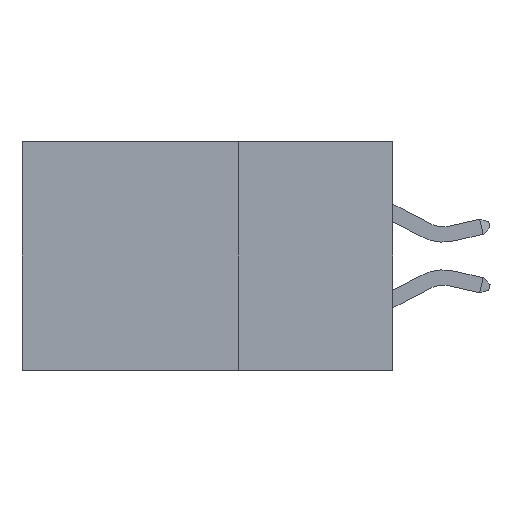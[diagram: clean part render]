
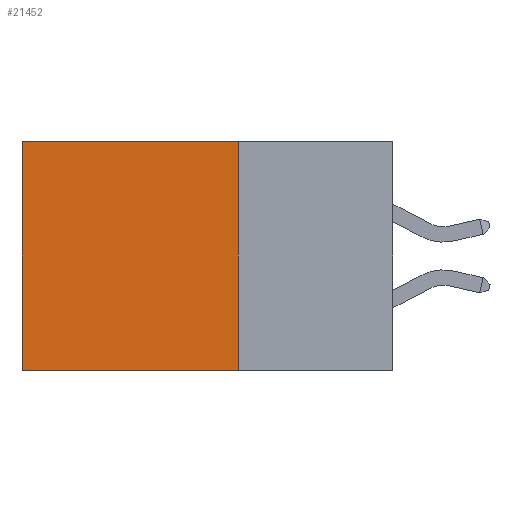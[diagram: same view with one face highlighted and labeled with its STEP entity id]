
A CAD part, left-side view. The second image highlights one B-rep face of the part: STEP entity #21452.
In plain terms, the highlighted planar face has unit normal (-1, 0, 0).
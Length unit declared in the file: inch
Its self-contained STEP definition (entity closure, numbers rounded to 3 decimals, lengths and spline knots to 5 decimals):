
#387 = LINE ( 'NONE', #5251, #19746 ) ;
#1677 = ORIENTED_EDGE ( 'NONE', *, *, #12777, .F. ) ;
#1767 = CARTESIAN_POINT ( 'NONE',  ( 0.2875, 0.6, 0. ) ) ;
#2341 = ORIENTED_EDGE ( 'NONE', *, *, #16443, .T. ) ;
#2818 = CARTESIAN_POINT ( 'NONE',  ( 0.2875, 0.6, -0.37 ) ) ;
#3862 = CARTESIAN_POINT ( 'NONE',  ( 0.2875, 0.25, 0. ) ) ;
#4780 = ORIENTED_EDGE ( 'NONE', *, *, #15298, .F. ) ;
#4854 = LINE ( 'NONE', #25881, #7781 ) ;
#5251 = CARTESIAN_POINT ( 'NONE',  ( 0.2875, 0.6, 0. ) ) ;
#6839 = FACE_OUTER_BOUND ( 'NONE', #13002, .T. ) ;
#7776 = DIRECTION ( 'NONE',  ( 1., 0., 0. ) ) ;
#7781 = VECTOR ( 'NONE', #17425, 39.37008 ) ;
#9532 = EDGE_CURVE ( 'NONE', #23064, #10732, #387, .T. ) ;
#10037 = VERTEX_POINT ( 'NONE', #19476 ) ;
#10732 = VERTEX_POINT ( 'NONE', #2818 ) ;
#10864 = CARTESIAN_POINT ( 'NONE',  ( 0.2875, 0.25, 0. ) ) ;
#12258 = AXIS2_PLACEMENT_3D ( 'NONE', #3862, #7776, #22147 ) ;
#12777 = EDGE_CURVE ( 'NONE', #10037, #20554, #4854, .T. ) ;
#13002 = EDGE_LOOP ( 'NONE', ( #22026, #4780, #1677, #2341 ) ) ;
#13224 = CARTESIAN_POINT ( 'NONE',  ( 0.2875, 0.25, -0.37 ) ) ;
#13560 = DIRECTION ( 'NONE',  ( 0., 0., -1. ) ) ;
#15065 = DIRECTION ( 'NONE',  ( 0., 1., 0. ) ) ;
#15298 = EDGE_CURVE ( 'NONE', #20554, #10732, #20516, .T. ) ;
#16443 = EDGE_CURVE ( 'NONE', #10037, #23064, #26598, .T. ) ;
#17425 = DIRECTION ( 'NONE',  ( 0., 0., -1. ) ) ;
#19476 = CARTESIAN_POINT ( 'NONE',  ( 0.2875, 0.25, 0. ) ) ;
#19746 = VECTOR ( 'NONE', #13560, 39.37008 ) ;
#20066 = PLANE ( 'NONE',  #12258 ) ;
#20516 = LINE ( 'NONE', #13224, #23100 ) ;
#20554 = VERTEX_POINT ( 'NONE', #26060 ) ;
#21452 = ADVANCED_FACE ( 'NONE', ( #6839 ), #20066, .F. ) ;
#22026 = ORIENTED_EDGE ( 'NONE', *, *, #9532, .T. ) ;
#22147 = DIRECTION ( 'NONE',  ( 0., 0., -1. ) ) ;
#22255 = DIRECTION ( 'NONE',  ( 0., 1., 0. ) ) ;
#23064 = VERTEX_POINT ( 'NONE', #1767 ) ;
#23100 = VECTOR ( 'NONE', #22255, 39.37008 ) ;
#23688 = VECTOR ( 'NONE', #15065, 39.37008 ) ;
#25881 = CARTESIAN_POINT ( 'NONE',  ( 0.2875, 0.25, 0. ) ) ;
#26060 = CARTESIAN_POINT ( 'NONE',  ( 0.2875, 0.25, -0.37 ) ) ;
#26598 = LINE ( 'NONE', #10864, #23688 ) ;
